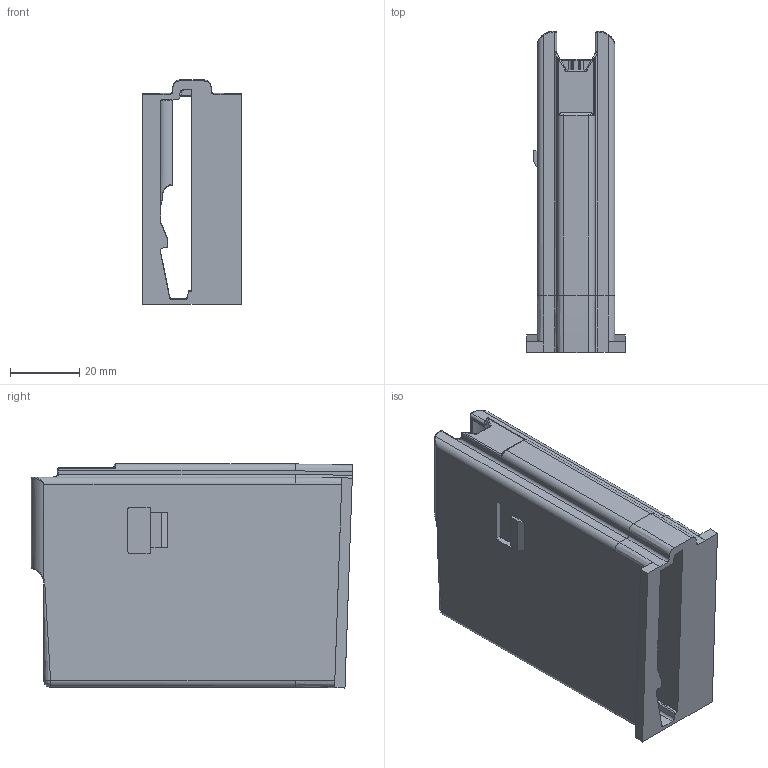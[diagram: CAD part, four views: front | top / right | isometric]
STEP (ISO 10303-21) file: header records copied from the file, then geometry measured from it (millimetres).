
FILE_DESCRIPTION (( 'STEP AP214' ), '1' );
FILE_NAME ('feed_lips.STEP', '2013-12-22T02:37:11', ( '' ), ( '' ), 'SwSTEP 2.0', 'SolidWorks 2013', '' );
FILE_SCHEMA (( 'AUTOMOTIVE_DESIGN' ));
Length unit declared in the file: millimetre
Products named in the file (1): feed_lips
Bounding box: 28.5 x 92.93 x 64.77 mm (x, y, z)
Volume: 76940.2 mm3; surface area: 29992.5 mm2
Topology: 1 solids, 1 shells, 285 faces, 711 edges, 414 vertices
Faces by surface type: bspline 114, cylinder 103, plane 65, cone 3
Entity records: 13203 total; most frequent: CARTESIAN_POINT 7323, ORIENTED_EDGE 1394, DIRECTION 1019, EDGE_CURVE 697, VERTEX_POINT 414, AXIS2_PLACEMENT_3D 373, EDGE_LOOP 287, FACE_OUTER_BOUND 285
